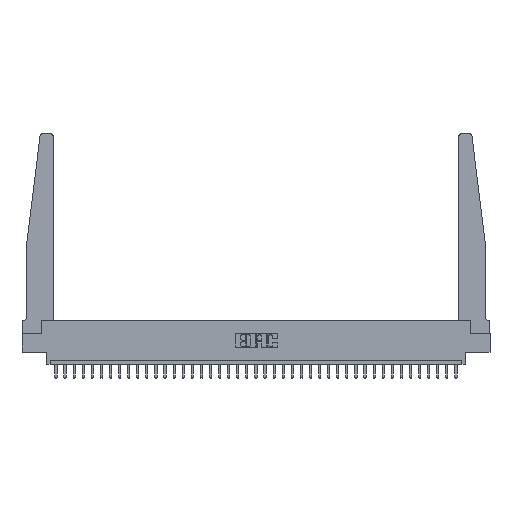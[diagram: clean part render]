
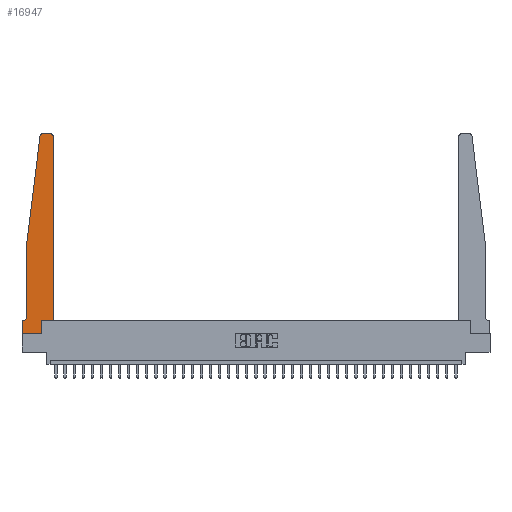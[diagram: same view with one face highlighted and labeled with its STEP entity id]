
A CAD part, top view. The second image highlights one B-rep face of the part: STEP entity #16947.
In plain terms, the highlighted planar face has unit normal (0, 0, 1).
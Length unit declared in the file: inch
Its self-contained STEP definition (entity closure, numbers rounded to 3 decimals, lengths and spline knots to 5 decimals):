
#157 = VECTOR ( 'NONE', #25622, 39.37008 ) ;
#390 = CARTESIAN_POINT ( 'NONE',  ( 0.25, 2.75, 0.37 ) ) ;
#498 = CARTESIAN_POINT ( 'NONE',  ( 0.27653, 2.72, 0.37 ) ) ;
#646 = LINE ( 'NONE', #13837, #20630 ) ;
#1016 = LINE ( 'NONE', #30894, #28649 ) ;
#1207 = EDGE_CURVE ( 'NONE', #27892, #22182, #16064, .T. ) ;
#1298 = CIRCLE ( 'NONE', #12512, 0.03 ) ;
#1753 = ORIENTED_EDGE ( 'NONE', *, *, #21778, .T. ) ;
#1926 = CARTESIAN_POINT ( 'NONE',  ( 0.015, 0.1875, 0.37 ) ) ;
#2284 = CARTESIAN_POINT ( 'NONE',  ( 0., 0.1875, 0.37 ) ) ;
#2320 = DIRECTION ( 'NONE',  ( 1., 0., 0. ) ) ;
#2410 = EDGE_CURVE ( 'NONE', #6980, #31797, #9356, .T. ) ;
#2466 = EDGE_CURVE ( 'NONE', #31797, #28150, #28752, .T. ) ;
#2634 = LINE ( 'NONE', #22831, #19055 ) ;
#2813 = VERTEX_POINT ( 'NONE', #16363 ) ;
#3144 = EDGE_CURVE ( 'NONE', #28150, #19034, #9840, .T. ) ;
#3331 = CARTESIAN_POINT ( 'NONE',  ( 0.2605, 0.18, 0.37 ) ) ;
#3684 = DIRECTION ( 'NONE',  ( 1., 0., 0. ) ) ;
#3819 = VECTOR ( 'NONE', #18890, 39.37008 ) ;
#4506 = AXIS2_PLACEMENT_3D ( 'NONE', #5013, #15200, #10690 ) ;
#4988 = CARTESIAN_POINT ( 'NONE',  ( 0., 0., 0.37 ) ) ;
#5013 = CARTESIAN_POINT ( 'NONE',  ( 0., 0.1875, 0.37 ) ) ;
#5586 = LINE ( 'NONE', #32945, #157 ) ;
#6155 = CARTESIAN_POINT ( 'NONE',  ( 0.425, 0.18, 0.37 ) ) ;
#6980 = VERTEX_POINT ( 'NONE', #12231 ) ;
#7320 = CARTESIAN_POINT ( 'NONE',  ( 0.395, 2.72, 0.37 ) ) ;
#8062 = CARTESIAN_POINT ( 'NONE',  ( 0., 0., 0.37 ) ) ;
#9356 = CIRCLE ( 'NONE', #12564, 0.05 ) ;
#9840 = LINE ( 'NONE', #4988, #19682 ) ;
#10312 = CIRCLE ( 'NONE', #23655, 0.03 ) ;
#10690 = DIRECTION ( 'NONE',  ( 1., 0., 0. ) ) ;
#10825 = ORIENTED_EDGE ( 'NONE', *, *, #1207, .T. ) ;
#11221 = CARTESIAN_POINT ( 'NONE',  ( 0.24675, 2.72367, 0.37 ) ) ;
#11777 = ORIENTED_EDGE ( 'NONE', *, *, #13383, .T. ) ;
#12032 = VERTEX_POINT ( 'NONE', #23706 ) ;
#12097 = EDGE_CURVE ( 'NONE', #2813, #17004, #31500, .T. ) ;
#12231 = CARTESIAN_POINT ( 'NONE',  ( 0.065, 0.2375, 0.37 ) ) ;
#12512 = AXIS2_PLACEMENT_3D ( 'NONE', #7320, #17501, #2320 ) ;
#12542 = FACE_OUTER_BOUND ( 'NONE', #27762, .T. ) ;
#12564 = AXIS2_PLACEMENT_3D ( 'NONE', #31076, #13741, #16068 ) ;
#12602 = ORIENTED_EDGE ( 'NONE', *, *, #22688, .T. ) ;
#12830 = DIRECTION ( 'NONE',  ( 1., 0., 0. ) ) ;
#12871 = VERTEX_POINT ( 'NONE', #11221 ) ;
#13383 = EDGE_CURVE ( 'NONE', #12032, #6980, #5586, .T. ) ;
#13741 = DIRECTION ( 'NONE',  ( 0., 0., -1. ) ) ;
#13782 = VECTOR ( 'NONE', #14295, 39.37008 ) ;
#13837 = CARTESIAN_POINT ( 'NONE',  ( 0.2605, 0.18, 0.37 ) ) ;
#14295 = DIRECTION ( 'NONE',  ( -0.122, -0.992, 0. ) ) ;
#15200 = DIRECTION ( 'NONE',  ( 0., 0., 1. ) ) ;
#15730 = EDGE_CURVE ( 'NONE', #22182, #12871, #10312, .T. ) ;
#15993 = ORIENTED_EDGE ( 'NONE', *, *, #21258, .T. ) ;
#16064 = LINE ( 'NONE', #390, #3819 ) ;
#16068 = DIRECTION ( 'NONE',  ( -1., 0., 0. ) ) ;
#16363 = CARTESIAN_POINT ( 'NONE',  ( 0.425, 0.18, 0.37 ) ) ;
#16833 = VECTOR ( 'NONE', #23585, 39.37008 ) ;
#16947 = ADVANCED_FACE ( 'NONE', ( #12542 ), #30372, .T. ) ;
#17004 = VERTEX_POINT ( 'NONE', #28546 ) ;
#17056 = VERTEX_POINT ( 'NONE', #3331 ) ;
#17501 = DIRECTION ( 'NONE',  ( 0., 0., 1. ) ) ;
#18847 = DIRECTION ( 'NONE',  ( 0., 1., 0. ) ) ;
#18890 = DIRECTION ( 'NONE',  ( -1., 0., 0. ) ) ;
#19025 = ORIENTED_EDGE ( 'NONE', *, *, #22378, .T. ) ;
#19034 = VERTEX_POINT ( 'NONE', #8062 ) ;
#19055 = VECTOR ( 'NONE', #12830, 39.37008 ) ;
#19165 = CARTESIAN_POINT ( 'NONE',  ( 0.27653, 2.75, 0.37 ) ) ;
#19682 = VECTOR ( 'NONE', #22854, 39.37008 ) ;
#19854 = ORIENTED_EDGE ( 'NONE', *, *, #2466, .T. ) ;
#20022 = ORIENTED_EDGE ( 'NONE', *, *, #12097, .T. ) ;
#20630 = VECTOR ( 'NONE', #29168, 39.37008 ) ;
#20645 = ORIENTED_EDGE ( 'NONE', *, *, #26631, .T. ) ;
#20819 = ORIENTED_EDGE ( 'NONE', *, *, #15730, .T. ) ;
#20858 = DIRECTION ( 'NONE',  ( 0., 0., 1. ) ) ;
#21014 = CARTESIAN_POINT ( 'NONE',  ( 0.395, 2.75, 0.37 ) ) ;
#21258 = EDGE_CURVE ( 'NONE', #29663, #17056, #646, .T. ) ;
#21778 = EDGE_CURVE ( 'NONE', #17056, #2813, #1016, .T. ) ;
#22182 = VERTEX_POINT ( 'NONE', #19165 ) ;
#22378 = EDGE_CURVE ( 'NONE', #19034, #29663, #2634, .T. ) ;
#22688 = EDGE_CURVE ( 'NONE', #12871, #12032, #31785, .T. ) ;
#22831 = CARTESIAN_POINT ( 'NONE',  ( 0., 0., 0.37 ) ) ;
#22854 = DIRECTION ( 'NONE',  ( 0., -1., 0. ) ) ;
#23554 = CARTESIAN_POINT ( 'NONE',  ( 0.2605, 0., 0.37 ) ) ;
#23585 = DIRECTION ( 'NONE',  ( -1., 0., 0. ) ) ;
#23655 = AXIS2_PLACEMENT_3D ( 'NONE', #498, #20858, #26031 ) ;
#23706 = CARTESIAN_POINT ( 'NONE',  ( 0.065, 1.25, 0.37 ) ) ;
#25622 = DIRECTION ( 'NONE',  ( 0., -1., 0. ) ) ;
#26031 = DIRECTION ( 'NONE',  ( 1., 0., 0. ) ) ;
#26241 = CARTESIAN_POINT ( 'NONE',  ( 0.065, 0.1875, 0.37 ) ) ;
#26480 = CARTESIAN_POINT ( 'NONE',  ( 0.065, 1.25, 0.37 ) ) ;
#26631 = EDGE_CURVE ( 'NONE', #17004, #27892, #1298, .T. ) ;
#27762 = EDGE_LOOP ( 'NONE', ( #10825, #20819, #12602, #11777, #28950, #19854, #31199, #19025, #15993, #1753, #20022, #20645 ) ) ;
#27892 = VERTEX_POINT ( 'NONE', #21014 ) ;
#28150 = VERTEX_POINT ( 'NONE', #2284 ) ;
#28546 = CARTESIAN_POINT ( 'NONE',  ( 0.425, 2.72, 0.37 ) ) ;
#28649 = VECTOR ( 'NONE', #3684, 39.37008 ) ;
#28752 = LINE ( 'NONE', #26241, #16833 ) ;
#28950 = ORIENTED_EDGE ( 'NONE', *, *, #2410, .T. ) ;
#29168 = DIRECTION ( 'NONE',  ( 0., 1., 0. ) ) ;
#29387 = VECTOR ( 'NONE', #18847, 39.37008 ) ;
#29663 = VERTEX_POINT ( 'NONE', #23554 ) ;
#30372 = PLANE ( 'NONE',  #4506 ) ;
#30894 = CARTESIAN_POINT ( 'NONE',  ( 0.425, 0.18, 0.37 ) ) ;
#31076 = CARTESIAN_POINT ( 'NONE',  ( 0.015, 0.2375, 0.37 ) ) ;
#31199 = ORIENTED_EDGE ( 'NONE', *, *, #3144, .T. ) ;
#31500 = LINE ( 'NONE', #6155, #29387 ) ;
#31785 = LINE ( 'NONE', #26480, #13782 ) ;
#31797 = VERTEX_POINT ( 'NONE', #1926 ) ;
#32945 = CARTESIAN_POINT ( 'NONE',  ( 0.065, 1.25, 0.37 ) ) ;
